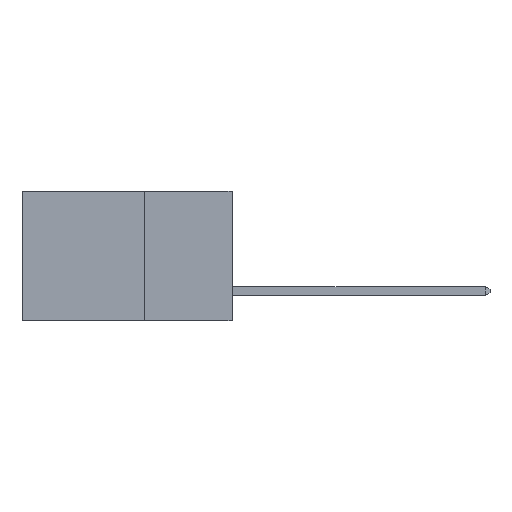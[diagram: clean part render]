
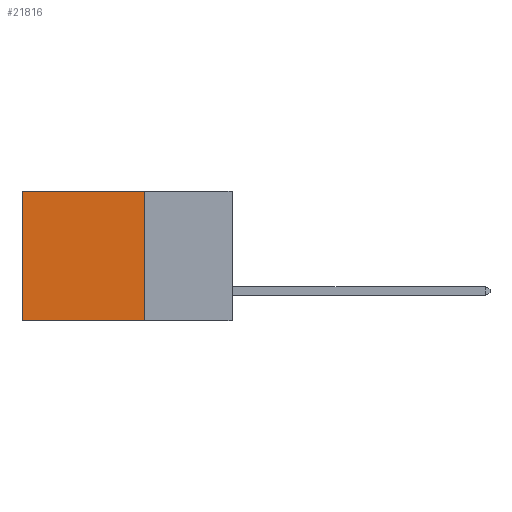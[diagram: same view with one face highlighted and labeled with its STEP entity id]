
A CAD part, left-side view. The second image highlights one B-rep face of the part: STEP entity #21816.
In plain terms, the highlighted planar face has unit normal (-1, 0, 0).
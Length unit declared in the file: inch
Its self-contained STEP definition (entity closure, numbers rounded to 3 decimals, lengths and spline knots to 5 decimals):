
#2155 = DIRECTION ( 'NONE',  ( 0., 0., -1. ) ) ;
#3123 = EDGE_CURVE ( 'NONE', #17366, #22151, #5770, .T. ) ;
#3485 = CARTESIAN_POINT ( 'NONE',  ( 0.2875, 0.25, -0.37 ) ) ;
#4949 = VECTOR ( 'NONE', #31446, 39.37008 ) ;
#5770 = LINE ( 'NONE', #11849, #11688 ) ;
#7038 = FACE_OUTER_BOUND ( 'NONE', #26043, .T. ) ;
#8219 = EDGE_CURVE ( 'NONE', #31844, #28916, #17758, .T. ) ;
#8374 = CARTESIAN_POINT ( 'NONE',  ( 0.2875, 0.25, 0. ) ) ;
#9690 = CARTESIAN_POINT ( 'NONE',  ( 0.2875, 0.25, 0. ) ) ;
#9713 = CARTESIAN_POINT ( 'NONE',  ( 0.2875, 0.6, 0. ) ) ;
#10265 = VECTOR ( 'NONE', #29803, 39.37008 ) ;
#11688 = VECTOR ( 'NONE', #26877, 39.37008 ) ;
#11849 = CARTESIAN_POINT ( 'NONE',  ( 0.2875, 0.25, 0. ) ) ;
#12451 = LINE ( 'NONE', #16422, #4949 ) ;
#12977 = CARTESIAN_POINT ( 'NONE',  ( 0.2875, 0.6, 0. ) ) ;
#13101 = ORIENTED_EDGE ( 'NONE', *, *, #8219, .T. ) ;
#13632 = AXIS2_PLACEMENT_3D ( 'NONE', #9690, #17294, #2155 ) ;
#14750 = PLANE ( 'NONE',  #13632 ) ;
#15453 = ORIENTED_EDGE ( 'NONE', *, *, #17356, .F. ) ;
#15843 = CARTESIAN_POINT ( 'NONE',  ( 0.2875, 0.25, -0.37 ) ) ;
#16422 = CARTESIAN_POINT ( 'NONE',  ( 0.2875, 0.25, 0. ) ) ;
#16873 = EDGE_CURVE ( 'NONE', #17366, #31844, #12451, .T. ) ;
#17210 = ORIENTED_EDGE ( 'NONE', *, *, #16873, .T. ) ;
#17294 = DIRECTION ( 'NONE',  ( 1., 0., 0. ) ) ;
#17356 = EDGE_CURVE ( 'NONE', #22151, #28916, #30097, .T. ) ;
#17366 = VERTEX_POINT ( 'NONE', #8374 ) ;
#17758 = LINE ( 'NONE', #9713, #10265 ) ;
#21816 = ADVANCED_FACE ( 'NONE', ( #7038 ), #14750, .F. ) ;
#22151 = VERTEX_POINT ( 'NONE', #3485 ) ;
#22447 = CARTESIAN_POINT ( 'NONE',  ( 0.2875, 0.6, -0.37 ) ) ;
#25407 = ORIENTED_EDGE ( 'NONE', *, *, #3123, .F. ) ;
#25933 = DIRECTION ( 'NONE',  ( 0., 1., 0. ) ) ;
#26043 = EDGE_LOOP ( 'NONE', ( #13101, #15453, #25407, #17210 ) ) ;
#26877 = DIRECTION ( 'NONE',  ( 0., 0., -1. ) ) ;
#28508 = VECTOR ( 'NONE', #25933, 39.37008 ) ;
#28916 = VERTEX_POINT ( 'NONE', #22447 ) ;
#29803 = DIRECTION ( 'NONE',  ( 0., 0., -1. ) ) ;
#30097 = LINE ( 'NONE', #15843, #28508 ) ;
#31446 = DIRECTION ( 'NONE',  ( 0., 1., 0. ) ) ;
#31844 = VERTEX_POINT ( 'NONE', #12977 ) ;
